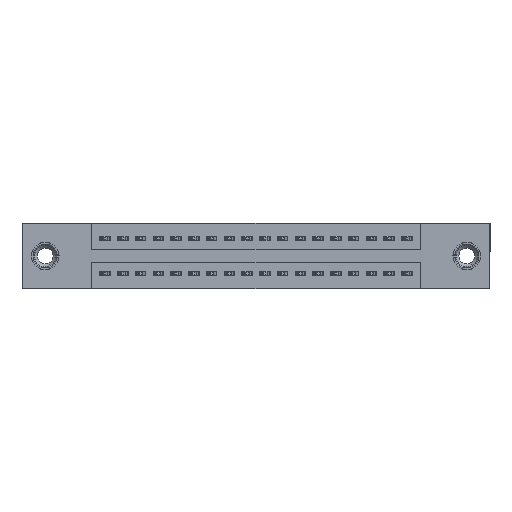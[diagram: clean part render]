
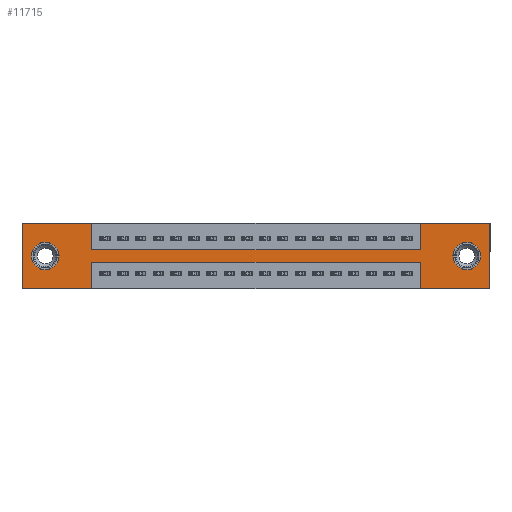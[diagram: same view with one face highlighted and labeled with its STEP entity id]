
A CAD part, front view. The second image highlights one B-rep face of the part: STEP entity #11715.
In plain terms, the highlighted planar face has unit normal (0, -1, 0).
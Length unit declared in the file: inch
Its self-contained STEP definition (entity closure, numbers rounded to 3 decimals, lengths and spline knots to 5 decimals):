
#125 = ORIENTED_EDGE ( 'NONE', *, *, #13101, .F. ) ;
#276 = CARTESIAN_POINT ( 'NONE',  ( 0.13, 0., -0.185 ) ) ;
#533 = ORIENTED_EDGE ( 'NONE', *, *, #16169, .T. ) ;
#593 = CARTESIAN_POINT ( 'NONE',  ( 0.3925, 0., -0.22 ) ) ;
#674 = DIRECTION ( 'NONE',  ( 0., 0., -1. ) ) ;
#675 = AXIS2_PLACEMENT_3D ( 'NONE', #17949, #8939, #19440 ) ;
#684 = CARTESIAN_POINT ( 'NONE',  ( 2.635, 0., 0. ) ) ;
#710 = ORIENTED_EDGE ( 'NONE', *, *, #10087, .F. ) ;
#1321 = VERTEX_POINT ( 'NONE', #17312 ) ;
#1602 = EDGE_LOOP ( 'NONE', ( #6036, #1765 ) ) ;
#1618 = FACE_BOUND ( 'NONE', #1602, .T. ) ;
#1765 = ORIENTED_EDGE ( 'NONE', *, *, #9670, .T. ) ;
#1769 = DIRECTION ( 'NONE',  ( 0., 0., 1. ) ) ;
#1774 = CARTESIAN_POINT ( 'NONE',  ( 0.13, 0., -0.185 ) ) ;
#1804 = ORIENTED_EDGE ( 'NONE', *, *, #12733, .T. ) ;
#1856 = VERTEX_POINT ( 'NONE', #10090 ) ;
#1890 = LINE ( 'NONE', #16927, #13074 ) ;
#1909 = VECTOR ( 'NONE', #674, 39.37008 ) ;
#2164 = VECTOR ( 'NONE', #9489, 39.37008 ) ;
#2176 = DIRECTION ( 'NONE',  ( 0., 0., -1. ) ) ;
#2446 = VERTEX_POINT ( 'NONE', #5243 ) ;
#2494 = VECTOR ( 'NONE', #6729, 39.37008 ) ;
#2541 = CARTESIAN_POINT ( 'NONE',  ( 0., 0., -0.37 ) ) ;
#2694 = CARTESIAN_POINT ( 'NONE',  ( 0., 0., -0.37 ) ) ;
#2866 = CARTESIAN_POINT ( 'NONE',  ( 0., 0., 0. ) ) ;
#2872 = VECTOR ( 'NONE', #8178, 39.37008 ) ;
#3298 = DIRECTION ( 'NONE',  ( 0., 0., 1. ) ) ;
#3387 = ORIENTED_EDGE ( 'NONE', *, *, #10586, .F. ) ;
#3407 = ORIENTED_EDGE ( 'NONE', *, *, #16785, .F. ) ;
#3438 = VECTOR ( 'NONE', #2176, 39.37008 ) ;
#3490 = DIRECTION ( 'NONE',  ( 0., 1., 0. ) ) ;
#3593 = CARTESIAN_POINT ( 'NONE',  ( 0.3925, 0., -0.37 ) ) ;
#3667 = EDGE_CURVE ( 'NONE', #19112, #18634, #6218, .T. ) ;
#3784 = CARTESIAN_POINT ( 'NONE',  ( 0.3925, 0., -0.22 ) ) ;
#4519 = CARTESIAN_POINT ( 'NONE',  ( 2.505, 0., -0.263 ) ) ;
#4674 = VERTEX_POINT ( 'NONE', #10579 ) ;
#4728 = CARTESIAN_POINT ( 'NONE',  ( 0., 0., 0. ) ) ;
#4866 = EDGE_CURVE ( 'NONE', #8337, #6829, #9058, .T. ) ;
#5019 = CARTESIAN_POINT ( 'NONE',  ( 0.3925, 0., -0.37 ) ) ;
#5243 = CARTESIAN_POINT ( 'NONE',  ( 2.2425, 0., -0.37 ) ) ;
#5570 = AXIS2_PLACEMENT_3D ( 'NONE', #276, #10877, #1769 ) ;
#5839 = LINE ( 'NONE', #4728, #13907 ) ;
#5897 = VERTEX_POINT ( 'NONE', #8592 ) ;
#5931 = ORIENTED_EDGE ( 'NONE', *, *, #5968, .F. ) ;
#5968 = EDGE_CURVE ( 'NONE', #7917, #2446, #14188, .T. ) ;
#6036 = ORIENTED_EDGE ( 'NONE', *, *, #4866, .T. ) ;
#6212 = ORIENTED_EDGE ( 'NONE', *, *, #3667, .F. ) ;
#6218 = LINE ( 'NONE', #18501, #2164 ) ;
#6340 = DIRECTION ( 'NONE',  ( 1., 0., 0. ) ) ;
#6729 = DIRECTION ( 'NONE',  ( 0., 0., 1. ) ) ;
#6829 = VERTEX_POINT ( 'NONE', #4519 ) ;
#7081 = VECTOR ( 'NONE', #13331, 39.37008 ) ;
#7099 = VECTOR ( 'NONE', #11980, 39.37008 ) ;
#7509 = ORIENTED_EDGE ( 'NONE', *, *, #15264, .F. ) ;
#7771 = ORIENTED_EDGE ( 'NONE', *, *, #16976, .F. ) ;
#7807 = DIRECTION ( 'NONE',  ( 0., 0., 1. ) ) ;
#7917 = VERTEX_POINT ( 'NONE', #17729 ) ;
#8146 = CARTESIAN_POINT ( 'NONE',  ( 2.635, 0., 0. ) ) ;
#8178 = DIRECTION ( 'NONE',  ( 0., 0., 1. ) ) ;
#8337 = VERTEX_POINT ( 'NONE', #12805 ) ;
#8592 = CARTESIAN_POINT ( 'NONE',  ( 0.13, 0., -0.263 ) ) ;
#8790 = ORIENTED_EDGE ( 'NONE', *, *, #14445, .F. ) ;
#8917 = CARTESIAN_POINT ( 'NONE',  ( 0., 0., 0. ) ) ;
#8939 = DIRECTION ( 'NONE',  ( 0., 1., 0. ) ) ;
#9058 = CIRCLE ( 'NONE', #13642, 0.078 ) ;
#9489 = DIRECTION ( 'NONE',  ( -1., 0., 0. ) ) ;
#9670 = EDGE_CURVE ( 'NONE', #6829, #8337, #13110, .T. ) ;
#10021 = LINE ( 'NONE', #14251, #1909 ) ;
#10063 = EDGE_CURVE ( 'NONE', #19493, #18764, #18502, .T. ) ;
#10068 = DIRECTION ( 'NONE',  ( 0., 0., -1. ) ) ;
#10087 = EDGE_CURVE ( 'NONE', #18692, #17288, #10021, .T. ) ;
#10090 = CARTESIAN_POINT ( 'NONE',  ( 2.2425, 0., -0.22 ) ) ;
#10294 = EDGE_LOOP ( 'NONE', ( #533, #1804 ) ) ;
#10303 = LINE ( 'NONE', #8917, #17832 ) ;
#10393 = CARTESIAN_POINT ( 'NONE',  ( 0.3925, 0., -0.15 ) ) ;
#10502 = ORIENTED_EDGE ( 'NONE', *, *, #15660, .F. ) ;
#10579 = CARTESIAN_POINT ( 'NONE',  ( 0.13, 0., -0.107 ) ) ;
#10586 = EDGE_CURVE ( 'NONE', #17288, #19493, #1890, .T. ) ;
#10619 = AXIS2_PLACEMENT_3D ( 'NONE', #14546, #19075, #10068 ) ;
#10877 = DIRECTION ( 'NONE',  ( 0., 1., 0. ) ) ;
#11104 = CIRCLE ( 'NONE', #5570, 0.078 ) ;
#11254 = EDGE_LOOP ( 'NONE', ( #17722, #8790, #7771, #5931, #10502, #7509, #18979, #3387, #710, #125, #3407, #6212 ) ) ;
#11527 = PLANE ( 'NONE',  #10619 ) ;
#11539 = VERTEX_POINT ( 'NONE', #8146 ) ;
#11715 = ADVANCED_FACE ( 'NONE', ( #1618, #17248, #13256 ), #11527, .T. ) ;
#11939 = DIRECTION ( 'NONE',  ( 1., 0., 0. ) ) ;
#11971 = CIRCLE ( 'NONE', #17828, 0.078 ) ;
#11980 = DIRECTION ( 'NONE',  ( 1., 0., 0. ) ) ;
#12091 = LINE ( 'NONE', #684, #3438 ) ;
#12108 = LINE ( 'NONE', #2866, #7099 ) ;
#12415 = DIRECTION ( 'NONE',  ( 0., 1., 0. ) ) ;
#12472 = VECTOR ( 'NONE', #14108, 39.37008 ) ;
#12610 = CARTESIAN_POINT ( 'NONE',  ( 2.505, 0., -0.185 ) ) ;
#12733 = EDGE_CURVE ( 'NONE', #5897, #4674, #11971, .T. ) ;
#12735 = DIRECTION ( 'NONE',  ( -1., 0., 0. ) ) ;
#12805 = CARTESIAN_POINT ( 'NONE',  ( 2.505, 0., -0.107 ) ) ;
#13074 = VECTOR ( 'NONE', #6340, 39.37008 ) ;
#13101 = EDGE_CURVE ( 'NONE', #1321, #18692, #10303, .T. ) ;
#13110 = CIRCLE ( 'NONE', #675, 0.078 ) ;
#13256 = FACE_OUTER_BOUND ( 'NONE', #11254, .T. ) ;
#13320 = CARTESIAN_POINT ( 'NONE',  ( 0.3925, 0., 0. ) ) ;
#13331 = DIRECTION ( 'NONE',  ( -1., 0., 0. ) ) ;
#13642 = AXIS2_PLACEMENT_3D ( 'NONE', #12610, #3490, #14113 ) ;
#13782 = VECTOR ( 'NONE', #12735, 39.37008 ) ;
#13907 = VECTOR ( 'NONE', #7807, 39.37008 ) ;
#14108 = DIRECTION ( 'NONE',  ( 0., 0., -1. ) ) ;
#14113 = DIRECTION ( 'NONE',  ( 0., 0., -1. ) ) ;
#14188 = LINE ( 'NONE', #2694, #7081 ) ;
#14251 = CARTESIAN_POINT ( 'NONE',  ( 0.3925, 0., 0. ) ) ;
#14283 = CARTESIAN_POINT ( 'NONE',  ( 2.2425, 0., -0.37 ) ) ;
#14445 = EDGE_CURVE ( 'NONE', #1856, #17049, #18257, .T. ) ;
#14546 = CARTESIAN_POINT ( 'NONE',  ( 0., 0., -0.37 ) ) ;
#14929 = CARTESIAN_POINT ( 'NONE',  ( 2.2425, 0., 0. ) ) ;
#15264 = EDGE_CURVE ( 'NONE', #18764, #11539, #12108, .T. ) ;
#15660 = EDGE_CURVE ( 'NONE', #11539, #7917, #12091, .T. ) ;
#15968 = LINE ( 'NONE', #5019, #12472 ) ;
#16169 = EDGE_CURVE ( 'NONE', #4674, #5897, #11104, .T. ) ;
#16785 = EDGE_CURVE ( 'NONE', #18634, #1321, #5839, .T. ) ;
#16927 = CARTESIAN_POINT ( 'NONE',  ( 0.3925, 0., -0.15 ) ) ;
#16976 = EDGE_CURVE ( 'NONE', #2446, #1856, #18145, .T. ) ;
#17049 = VERTEX_POINT ( 'NONE', #3784 ) ;
#17248 = FACE_BOUND ( 'NONE', #10294, .T. ) ;
#17288 = VERTEX_POINT ( 'NONE', #10393 ) ;
#17312 = CARTESIAN_POINT ( 'NONE',  ( 0., 0., 0. ) ) ;
#17722 = ORIENTED_EDGE ( 'NONE', *, *, #18360, .F. ) ;
#17729 = CARTESIAN_POINT ( 'NONE',  ( 2.635, 0., -0.37 ) ) ;
#17828 = AXIS2_PLACEMENT_3D ( 'NONE', #1774, #12415, #3298 ) ;
#17832 = VECTOR ( 'NONE', #11939, 39.37008 ) ;
#17949 = CARTESIAN_POINT ( 'NONE',  ( 2.505, 0., -0.185 ) ) ;
#18145 = LINE ( 'NONE', #14283, #2494 ) ;
#18257 = LINE ( 'NONE', #593, #13782 ) ;
#18360 = EDGE_CURVE ( 'NONE', #17049, #19112, #15968, .T. ) ;
#18501 = CARTESIAN_POINT ( 'NONE',  ( 0., 0., -0.37 ) ) ;
#18502 = LINE ( 'NONE', #18726, #2872 ) ;
#18634 = VERTEX_POINT ( 'NONE', #2541 ) ;
#18692 = VERTEX_POINT ( 'NONE', #13320 ) ;
#18726 = CARTESIAN_POINT ( 'NONE',  ( 2.2425, 0., 0. ) ) ;
#18764 = VERTEX_POINT ( 'NONE', #14929 ) ;
#18979 = ORIENTED_EDGE ( 'NONE', *, *, #10063, .F. ) ;
#19075 = DIRECTION ( 'NONE',  ( 0., -1., 0. ) ) ;
#19112 = VERTEX_POINT ( 'NONE', #3593 ) ;
#19440 = DIRECTION ( 'NONE',  ( 0., 0., -1. ) ) ;
#19493 = VERTEX_POINT ( 'NONE', #19516 ) ;
#19516 = CARTESIAN_POINT ( 'NONE',  ( 2.2425, 0., -0.15 ) ) ;
